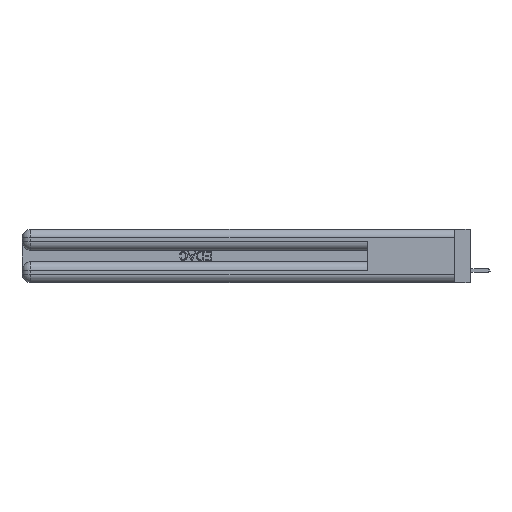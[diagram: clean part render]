
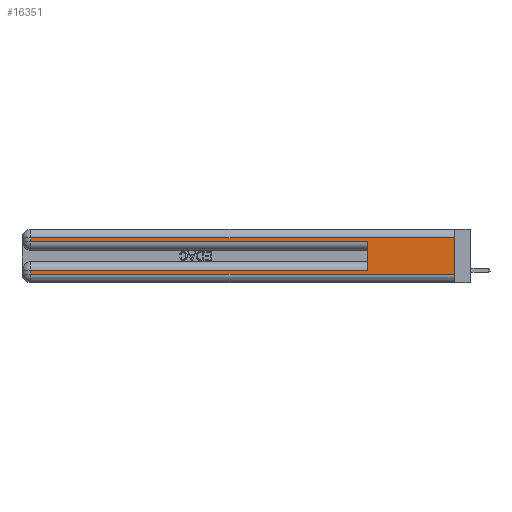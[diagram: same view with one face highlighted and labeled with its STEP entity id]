
A CAD part, left-side view. The second image highlights one B-rep face of the part: STEP entity #16351.
In plain terms, the highlighted planar face has unit normal (-1, 0, 0).
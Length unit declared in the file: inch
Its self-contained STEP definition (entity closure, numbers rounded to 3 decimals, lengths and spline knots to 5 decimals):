
#197 = ORIENTED_EDGE ( 'NONE', *, *, #29291, .T. ) ;
#374 = EDGE_CURVE ( 'NONE', #10527, #37095, #18474, .T. ) ;
#724 = VECTOR ( 'NONE', #39239, 39.37008 ) ;
#1041 = CARTESIAN_POINT ( 'NONE',  ( 0., 0., 0.06 ) ) ;
#2217 = DIRECTION ( 'NONE',  ( 0., -1., 0. ) ) ;
#5739 = VERTEX_POINT ( 'NONE', #11018 ) ;
#8460 = ORIENTED_EDGE ( 'NONE', *, *, #28985, .T. ) ;
#8577 = CARTESIAN_POINT ( 'NONE',  ( 0., 0., 0.285 ) ) ;
#8925 = DIRECTION ( 'NONE',  ( 0., 0., -1. ) ) ;
#9542 = VERTEX_POINT ( 'NONE', #47920 ) ;
#9552 = CARTESIAN_POINT ( 'NONE',  ( 0., 0., 0.37 ) ) ;
#10527 = VERTEX_POINT ( 'NONE', #11599 ) ;
#11018 = CARTESIAN_POINT ( 'NONE',  ( 0., 0., 0.06 ) ) ;
#11468 = ORIENTED_EDGE ( 'NONE', *, *, #16312, .F. ) ;
#11599 = CARTESIAN_POINT ( 'NONE',  ( 0., 0.6, 0.085 ) ) ;
#12074 = CARTESIAN_POINT ( 'NONE',  ( 0., 2.94, 0.06 ) ) ;
#12508 = VECTOR ( 'NONE', #43060, 39.37008 ) ;
#12807 = VERTEX_POINT ( 'NONE', #27459 ) ;
#15620 = DIRECTION ( 'NONE',  ( 0., 0., 1. ) ) ;
#16146 = VERTEX_POINT ( 'NONE', #12074 ) ;
#16312 = EDGE_CURVE ( 'NONE', #12807, #5739, #21201, .T. ) ;
#16336 = CARTESIAN_POINT ( 'NONE',  ( 0., 0.6, 0.145 ) ) ;
#16351 = ADVANCED_FACE ( 'NONE', ( #30746 ), #31269, .F. ) ;
#16433 = DIRECTION ( 'NONE',  ( 0., 0., -1. ) ) ;
#16790 = CARTESIAN_POINT ( 'NONE',  ( 0., 2.94, 0.37 ) ) ;
#16970 = DIRECTION ( 'NONE',  ( 0., 1., 0. ) ) ;
#17187 = EDGE_LOOP ( 'NONE', ( #11468, #38819, #27964, #8460, #29479, #197, #29959, #36022 ) ) ;
#17910 = DIRECTION ( 'NONE',  ( 0., 0., -1. ) ) ;
#18128 = DIRECTION ( 'NONE',  ( 1., 0., 0. ) ) ;
#18474 = LINE ( 'NONE', #16336, #43420 ) ;
#19917 = VECTOR ( 'NONE', #8925, 39.37008 ) ;
#21127 = LINE ( 'NONE', #16790, #22367 ) ;
#21201 = LINE ( 'NONE', #9552, #47400 ) ;
#21803 = CARTESIAN_POINT ( 'NONE',  ( 0., 2.94, 0.285 ) ) ;
#22367 = VECTOR ( 'NONE', #16433, 39.37008 ) ;
#22584 = VECTOR ( 'NONE', #2217, 39.37008 ) ;
#22599 = CARTESIAN_POINT ( 'NONE',  ( 0., 2.94, 0.085 ) ) ;
#23721 = EDGE_CURVE ( 'NONE', #46841, #16146, #31255, .T. ) ;
#23773 = CARTESIAN_POINT ( 'NONE',  ( 0., 0., 0.37 ) ) ;
#25536 = VECTOR ( 'NONE', #16970, 39.37008 ) ;
#27459 = CARTESIAN_POINT ( 'NONE',  ( 0., 0., 0.31 ) ) ;
#27964 = ORIENTED_EDGE ( 'NONE', *, *, #37161, .T. ) ;
#28985 = EDGE_CURVE ( 'NONE', #36023, #37095, #33891, .T. ) ;
#29162 = DIRECTION ( 'NONE',  ( 0., 0., -1. ) ) ;
#29291 = EDGE_CURVE ( 'NONE', #10527, #46841, #34993, .T. ) ;
#29479 = ORIENTED_EDGE ( 'NONE', *, *, #374, .F. ) ;
#29959 = ORIENTED_EDGE ( 'NONE', *, *, #23721, .T. ) ;
#30746 = FACE_OUTER_BOUND ( 'NONE', #17187, .T. ) ;
#31255 = LINE ( 'NONE', #31763, #19917 ) ;
#31269 = PLANE ( 'NONE',  #32740 ) ;
#31763 = CARTESIAN_POINT ( 'NONE',  ( 0., 2.94, 0.37 ) ) ;
#32740 = AXIS2_PLACEMENT_3D ( 'NONE', #23773, #18128, #29162 ) ;
#33891 = LINE ( 'NONE', #8577, #22584 ) ;
#34993 = LINE ( 'NONE', #43950, #25536 ) ;
#35608 = CARTESIAN_POINT ( 'NONE',  ( 0., 0., 0.31 ) ) ;
#36022 = ORIENTED_EDGE ( 'NONE', *, *, #47632, .T. ) ;
#36023 = VERTEX_POINT ( 'NONE', #21803 ) ;
#37095 = VERTEX_POINT ( 'NONE', #39101 ) ;
#37161 = EDGE_CURVE ( 'NONE', #9542, #36023, #21127, .T. ) ;
#38819 = ORIENTED_EDGE ( 'NONE', *, *, #38947, .T. ) ;
#38947 = EDGE_CURVE ( 'NONE', #12807, #9542, #41765, .T. ) ;
#39101 = CARTESIAN_POINT ( 'NONE',  ( 0., 0.6, 0.285 ) ) ;
#39239 = DIRECTION ( 'NONE',  ( 0., -1., 0. ) ) ;
#41383 = LINE ( 'NONE', #1041, #724 ) ;
#41765 = LINE ( 'NONE', #35608, #12508 ) ;
#43060 = DIRECTION ( 'NONE',  ( 0., 1., 0. ) ) ;
#43420 = VECTOR ( 'NONE', #15620, 39.37008 ) ;
#43950 = CARTESIAN_POINT ( 'NONE',  ( 0., 0., 0.085 ) ) ;
#46841 = VERTEX_POINT ( 'NONE', #22599 ) ;
#47400 = VECTOR ( 'NONE', #17910, 39.37008 ) ;
#47632 = EDGE_CURVE ( 'NONE', #16146, #5739, #41383, .T. ) ;
#47920 = CARTESIAN_POINT ( 'NONE',  ( 0., 2.94, 0.31 ) ) ;
